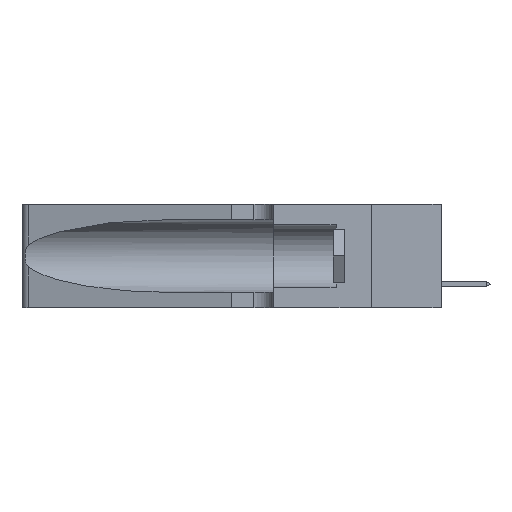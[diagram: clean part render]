
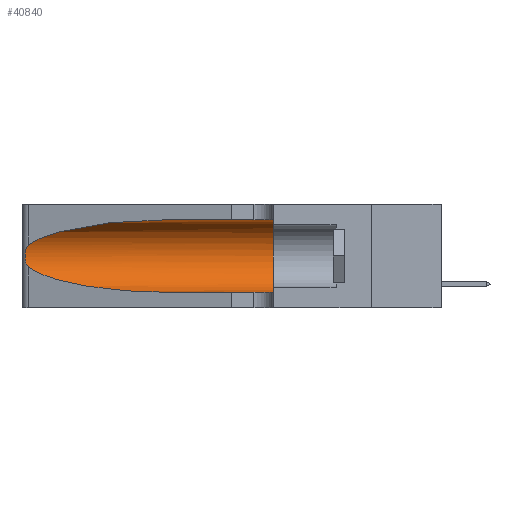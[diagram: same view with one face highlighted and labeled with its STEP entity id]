
A CAD part, left-side view. The second image highlights one B-rep face of the part: STEP entity #40840.
In plain terms, the highlighted cylindrical face has radius 3.308 mm (diameter 6.617 mm), a partial arc.
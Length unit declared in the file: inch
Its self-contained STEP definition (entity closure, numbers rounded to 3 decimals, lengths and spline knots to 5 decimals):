
#374 =( BOUNDED_CURVE ( )  B_SPLINE_CURVE ( 3, ( #7190, #49736, #43854, #1517 ),
 .UNSPECIFIED., .F., .F. ) 
 B_SPLINE_CURVE_WITH_KNOTS ( ( 4, 4 ),
 ( 1.5708, 2.84003 ),
 .UNSPECIFIED. ) 
 CURVE ( )  GEOMETRIC_REPRESENTATION_ITEM ( )  RATIONAL_B_SPLINE_CURVE ( ( 1., 0.87, 0.87, 1. ) ) 
 REPRESENTATION_ITEM ( '' )  );
#392 = CARTESIAN_POINT ( 'NONE',  ( 0.1305, 1.61858, 0.05475 ) ) ;
#638 = LINE ( 'NONE', #22128, #30303 ) ;
#1517 = CARTESIAN_POINT ( 'NONE',  ( 0.25487, 1.22718, 0.22369 ) ) ;
#3615 = ORIENTED_EDGE ( 'NONE', *, *, #44936, .T. ) ;
#4127 = B_SPLINE_CURVE_WITH_KNOTS ( 'NONE', 3,
 ( #29291, #10214, #36473, #29112, #33174, #10028, #13381, #40924, #30487, #32580, #47839, #19793, #20600, #36031 ),
 .UNSPECIFIED., .F., .F.,
 ( 4, 2, 2, 2, 2, 2, 4 ),
 ( 0., 0.00027, 0.00053, 0.00107, 0.0016, 0.00187, 0.00214 ),
 .UNSPECIFIED. ) ;
#6430 = CARTESIAN_POINT ( 'NONE',  ( 0.1305, 0.35, 0.31525 ) ) ;
#6769 = VERTEX_POINT ( 'NONE', #17885 ) ;
#7190 = CARTESIAN_POINT ( 'NONE',  ( 0.1305, 0.72297, 0.31525 ) ) ;
#7755 = FACE_OUTER_BOUND ( 'NONE', #43490, .T. ) ;
#8204 = EDGE_CURVE ( 'NONE', #37329, #20922, #16051, .T. ) ;
#8297 = EDGE_CURVE ( 'NONE', #6769, #19147, #638, .T. ) ;
#9711 = CARTESIAN_POINT ( 'NONE',  ( 0.1305, 0.72297, 0.05475 ) ) ;
#10028 = CARTESIAN_POINT ( 'NONE',  ( 0.26018, 1.23835, 0.19895 ) ) ;
#10214 = CARTESIAN_POINT ( 'NONE',  ( 0.25555, 1.22994, 0.2215 ) ) ;
#12745 = ORIENTED_EDGE ( 'NONE', *, *, #24311, .T. ) ;
#13381 = CARTESIAN_POINT ( 'NONE',  ( 0.26075, 1.23896, 0.19203 ) ) ;
#15219 = DIRECTION ( 'NONE',  ( 0., 0., 1. ) ) ;
#15961 = DIRECTION ( 'NONE',  ( 0., -1., 0. ) ) ;
#16051 =( BOUNDED_CURVE ( )  B_SPLINE_CURVE ( 3, ( #36168, #28777, #48372, #9711 ),
 .UNSPECIFIED., .F., .T. ) 
 B_SPLINE_CURVE_WITH_KNOTS ( ( 4, 4 ),
 ( 3.44316, 4.71239 ),
 .UNSPECIFIED. ) 
 CURVE ( )  GEOMETRIC_REPRESENTATION_ITEM ( )  RATIONAL_B_SPLINE_CURVE ( ( 1., 0.87, 0.87, 1. ) ) 
 REPRESENTATION_ITEM ( '' )  );
#17048 = VERTEX_POINT ( 'NONE', #41729 ) ;
#17717 = CARTESIAN_POINT ( 'NONE',  ( 0.1305, 0.35, 0.185 ) ) ;
#17885 = CARTESIAN_POINT ( 'NONE',  ( 0.1305, 0.72297, 0.31525 ) ) ;
#19147 = VERTEX_POINT ( 'NONE', #6430 ) ;
#19793 = CARTESIAN_POINT ( 'NONE',  ( 0.25639, 1.23186, 0.15144 ) ) ;
#20600 = CARTESIAN_POINT ( 'NONE',  ( 0.25555, 1.22993, 0.14849 ) ) ;
#20922 = VERTEX_POINT ( 'NONE', #48439 ) ;
#21649 = DIRECTION ( 'NONE',  ( 0., 1., 0. ) ) ;
#22128 = CARTESIAN_POINT ( 'NONE',  ( 0.1305, 1.61858, 0.31525 ) ) ;
#23672 = DIRECTION ( 'NONE',  ( 0., -1., 0. ) ) ;
#24048 = VECTOR ( 'NONE', #23672, 39.37008 ) ;
#24311 = EDGE_CURVE ( 'NONE', #6769, #17048, #374, .T. ) ;
#27061 = ORIENTED_EDGE ( 'NONE', *, *, #32111, .F. ) ;
#27112 = CYLINDRICAL_SURFACE ( 'NONE', #44742, 0.13025 ) ;
#28139 = DIRECTION ( 'NONE',  ( 0., 0., -1. ) ) ;
#28777 = CARTESIAN_POINT ( 'NONE',  ( 0.2373, 1.15595, 0.08982 ) ) ;
#29112 = CARTESIAN_POINT ( 'NONE',  ( 0.25787, 1.23484, 0.2124 ) ) ;
#29291 = CARTESIAN_POINT ( 'NONE',  ( 0.25487, 1.22718, 0.22369 ) ) ;
#30303 = VECTOR ( 'NONE', #30731, 39.37008 ) ;
#30487 = CARTESIAN_POINT ( 'NONE',  ( 0.26017, 1.23833, 0.17102 ) ) ;
#30731 = DIRECTION ( 'NONE',  ( 0., -1., 0. ) ) ;
#31270 = LINE ( 'NONE', #392, #24048 ) ;
#32111 = EDGE_CURVE ( 'NONE', #19147, #38042, #35556, .T. ) ;
#32126 = CARTESIAN_POINT ( 'NONE',  ( 0.25487, 1.22718, 0.14631 ) ) ;
#32516 = CARTESIAN_POINT ( 'NONE',  ( 0.1305, 0.35, 0.05475 ) ) ;
#32580 = CARTESIAN_POINT ( 'NONE',  ( 0.25856, 1.23593, 0.16098 ) ) ;
#33174 = CARTESIAN_POINT ( 'NONE',  ( 0.25854, 1.2359, 0.20912 ) ) ;
#34466 = EDGE_CURVE ( 'NONE', #17048, #37329, #4127, .T. ) ;
#35556 = CIRCLE ( 'NONE', #45654, 0.13025 ) ;
#36031 = CARTESIAN_POINT ( 'NONE',  ( 0.25487, 1.22718, 0.14631 ) ) ;
#36168 = CARTESIAN_POINT ( 'NONE',  ( 0.25487, 1.22718, 0.14631 ) ) ;
#36473 = CARTESIAN_POINT ( 'NONE',  ( 0.25639, 1.23184, 0.21858 ) ) ;
#37329 = VERTEX_POINT ( 'NONE', #32126 ) ;
#38042 = VERTEX_POINT ( 'NONE', #32516 ) ;
#39669 = ORIENTED_EDGE ( 'NONE', *, *, #8204, .T. ) ;
#40840 = ADVANCED_FACE ( 'NONE', ( #7755 ), #27112, .F. ) ;
#40924 = CARTESIAN_POINT ( 'NONE',  ( 0.26075, 1.23896, 0.178 ) ) ;
#41729 = CARTESIAN_POINT ( 'NONE',  ( 0.25487, 1.22718, 0.22369 ) ) ;
#43490 = EDGE_LOOP ( 'NONE', ( #12745, #47404, #39669, #3615, #27061, #43653 ) ) ;
#43653 = ORIENTED_EDGE ( 'NONE', *, *, #8297, .F. ) ;
#43854 = CARTESIAN_POINT ( 'NONE',  ( 0.2373, 1.15595, 0.28018 ) ) ;
#44742 = AXIS2_PLACEMENT_3D ( 'NONE', #45801, #15961, #28139 ) ;
#44936 = EDGE_CURVE ( 'NONE', #20922, #38042, #31270, .T. ) ;
#45654 = AXIS2_PLACEMENT_3D ( 'NONE', #17717, #21649, #15219 ) ;
#45801 = CARTESIAN_POINT ( 'NONE',  ( 0.1305, 1.61858, 0.185 ) ) ;
#47404 = ORIENTED_EDGE ( 'NONE', *, *, #34466, .T. ) ;
#47839 = CARTESIAN_POINT ( 'NONE',  ( 0.25789, 1.23486, 0.15765 ) ) ;
#48372 = CARTESIAN_POINT ( 'NONE',  ( 0.18966, 0.96281, 0.05475 ) ) ;
#48439 = CARTESIAN_POINT ( 'NONE',  ( 0.1305, 0.72297, 0.05475 ) ) ;
#49736 = CARTESIAN_POINT ( 'NONE',  ( 0.18966, 0.96281, 0.31525 ) ) ;
